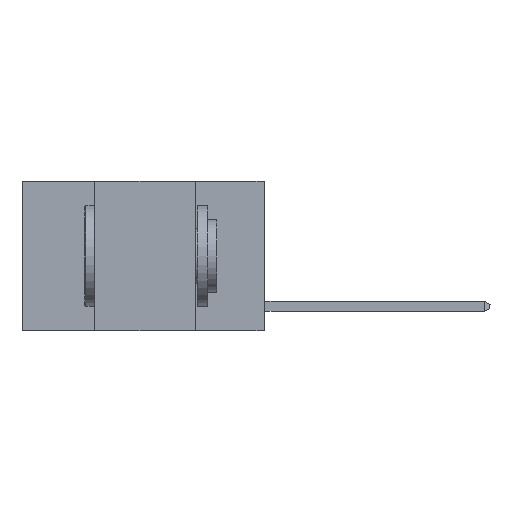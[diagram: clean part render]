
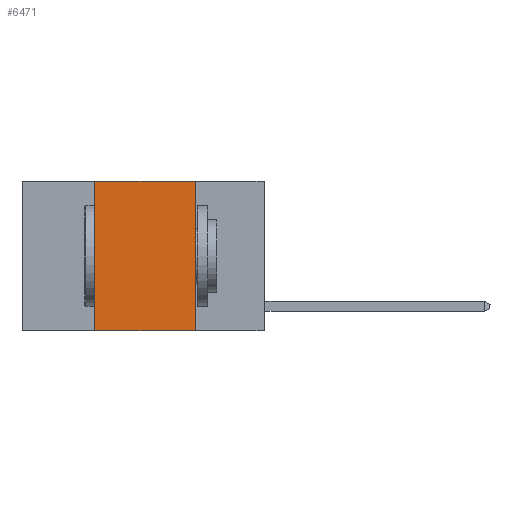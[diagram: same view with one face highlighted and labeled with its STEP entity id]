
A CAD part, left-side view. The second image highlights one B-rep face of the part: STEP entity #6471.
In plain terms, the highlighted planar face has unit normal (-1, 0, 0).
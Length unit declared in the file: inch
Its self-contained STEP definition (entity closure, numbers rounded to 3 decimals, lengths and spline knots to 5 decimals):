
#358 = LINE ( 'NONE', #12647, #3460 ) ;
#656 = DIRECTION ( 'NONE',  ( 0., -1., 0. ) ) ;
#819 = EDGE_CURVE ( 'NONE', #12896, #8089, #358, .T. ) ;
#1510 = ORIENTED_EDGE ( 'NONE', *, *, #819, .T. ) ;
#1511 = CARTESIAN_POINT ( 'NONE',  ( 0., 0.42, 0. ) ) ;
#2499 = LINE ( 'NONE', #12267, #8187 ) ;
#3326 = EDGE_CURVE ( 'NONE', #12896, #5832, #10463, .T. ) ;
#3460 = VECTOR ( 'NONE', #9122, 39.37008 ) ;
#3689 = EDGE_CURVE ( 'NONE', #10421, #8089, #2499, .T. ) ;
#4502 = PLANE ( 'NONE',  #10836 ) ;
#4843 = VECTOR ( 'NONE', #8317, 39.37008 ) ;
#4887 = CARTESIAN_POINT ( 'NONE',  ( 0., 0.17, -0.37 ) ) ;
#5625 = CARTESIAN_POINT ( 'NONE',  ( 0., 0.6, 0. ) ) ;
#5832 = VERTEX_POINT ( 'NONE', #11257 ) ;
#6129 = ORIENTED_EDGE ( 'NONE', *, *, #3689, .F. ) ;
#6471 = ADVANCED_FACE ( 'NONE', ( #11064 ), #4502, .F. ) ;
#6566 = EDGE_LOOP ( 'NONE', ( #6129, #12461, #9820, #1510 ) ) ;
#6674 = DIRECTION ( 'NONE',  ( 0., 0., -1. ) ) ;
#6785 = DIRECTION ( 'NONE',  ( 1., 0., 0. ) ) ;
#6808 = CARTESIAN_POINT ( 'NONE',  ( 0., 0.42, -0.37 ) ) ;
#7320 = VECTOR ( 'NONE', #656, 39.37008 ) ;
#8089 = VERTEX_POINT ( 'NONE', #4887 ) ;
#8187 = VECTOR ( 'NONE', #6674, 39.37008 ) ;
#8317 = DIRECTION ( 'NONE',  ( 0., 0., 1. ) ) ;
#8992 = EDGE_CURVE ( 'NONE', #5832, #10421, #12917, .T. ) ;
#9122 = DIRECTION ( 'NONE',  ( 0., -1., 0. ) ) ;
#9820 = ORIENTED_EDGE ( 'NONE', *, *, #3326, .F. ) ;
#10421 = VERTEX_POINT ( 'NONE', #14700 ) ;
#10463 = LINE ( 'NONE', #1511, #4843 ) ;
#10836 = AXIS2_PLACEMENT_3D ( 'NONE', #5625, #6785, #14608 ) ;
#11064 = FACE_OUTER_BOUND ( 'NONE', #6566, .T. ) ;
#11257 = CARTESIAN_POINT ( 'NONE',  ( 0., 0.42, 0. ) ) ;
#12267 = CARTESIAN_POINT ( 'NONE',  ( 0., 0.17, 0. ) ) ;
#12461 = ORIENTED_EDGE ( 'NONE', *, *, #8992, .F. ) ;
#12647 = CARTESIAN_POINT ( 'NONE',  ( 0., 0.6, -0.37 ) ) ;
#12896 = VERTEX_POINT ( 'NONE', #6808 ) ;
#12917 = LINE ( 'NONE', #14283, #7320 ) ;
#14283 = CARTESIAN_POINT ( 'NONE',  ( 0., 0.6, 0. ) ) ;
#14608 = DIRECTION ( 'NONE',  ( 0., 0., -1. ) ) ;
#14700 = CARTESIAN_POINT ( 'NONE',  ( 0., 0.17, 0. ) ) ;
